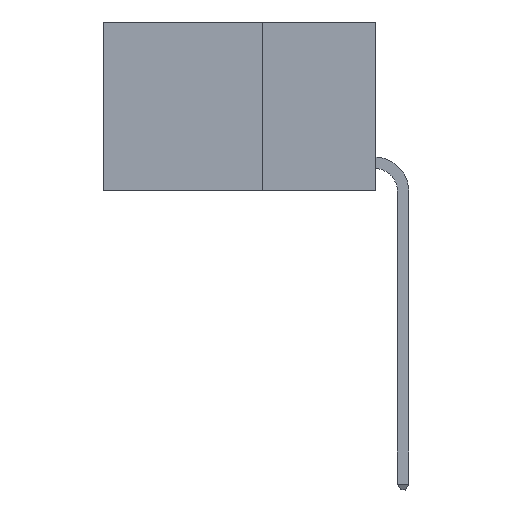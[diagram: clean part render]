
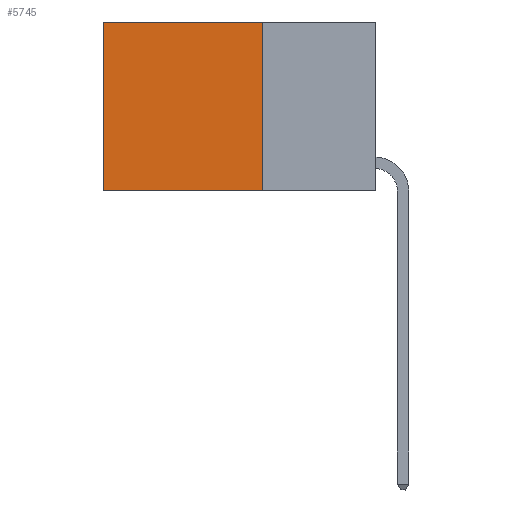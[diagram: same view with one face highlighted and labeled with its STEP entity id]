
A CAD part, left-side view. The second image highlights one B-rep face of the part: STEP entity #5745.
In plain terms, the highlighted planar face has unit normal (-1, 0, 0).
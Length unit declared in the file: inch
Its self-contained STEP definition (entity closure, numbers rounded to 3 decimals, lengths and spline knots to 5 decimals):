
#638 = CARTESIAN_POINT ( 'NONE',  ( 0.2625, 0.6, -0.37 ) ) ;
#828 = VECTOR ( 'NONE', #23020, 39.37008 ) ;
#937 = DIRECTION ( 'NONE',  ( 1., 0., 0. ) ) ;
#1519 = ORIENTED_EDGE ( 'NONE', *, *, #14590, .T. ) ;
#1627 = CARTESIAN_POINT ( 'NONE',  ( 0.2625, 0.25, 0. ) ) ;
#3688 = CARTESIAN_POINT ( 'NONE',  ( 0.2625, 0.25, 0. ) ) ;
#4303 = VECTOR ( 'NONE', #25474, 39.37008 ) ;
#4760 = EDGE_CURVE ( 'NONE', #25653, #25745, #23488, .T. ) ;
#5031 = DIRECTION ( 'NONE',  ( 0., 0., -1. ) ) ;
#5745 = ADVANCED_FACE ( 'NONE', ( #12976 ), #11008, .F. ) ;
#6198 = VERTEX_POINT ( 'NONE', #3688 ) ;
#7542 = CARTESIAN_POINT ( 'NONE',  ( 0.2625, 0.6, 0. ) ) ;
#8043 = VECTOR ( 'NONE', #16398, 39.37008 ) ;
#8261 = EDGE_CURVE ( 'NONE', #6198, #25653, #24998, .T. ) ;
#8448 = EDGE_CURVE ( 'NONE', #6198, #22909, #19741, .T. ) ;
#9805 = DIRECTION ( 'NONE',  ( 0., 0., -1. ) ) ;
#11008 = PLANE ( 'NONE',  #14078 ) ;
#12976 = FACE_OUTER_BOUND ( 'NONE', #14661, .T. ) ;
#13114 = ORIENTED_EDGE ( 'NONE', *, *, #8448, .T. ) ;
#13329 = CARTESIAN_POINT ( 'NONE',  ( 0.2625, 0.6, 0. ) ) ;
#14078 = AXIS2_PLACEMENT_3D ( 'NONE', #14698, #937, #5031 ) ;
#14590 = EDGE_CURVE ( 'NONE', #22909, #25745, #25600, .T. ) ;
#14661 = EDGE_LOOP ( 'NONE', ( #1519, #25498, #24419, #13114 ) ) ;
#14698 = CARTESIAN_POINT ( 'NONE',  ( 0.2625, 0.25, 0. ) ) ;
#15005 = CARTESIAN_POINT ( 'NONE',  ( 0.2625, 0.25, 0. ) ) ;
#15882 = CARTESIAN_POINT ( 'NONE',  ( 0.2625, 0.25, -0.37 ) ) ;
#16398 = DIRECTION ( 'NONE',  ( 0., 1., 0. ) ) ;
#17325 = CARTESIAN_POINT ( 'NONE',  ( 0.2625, 0.25, -0.37 ) ) ;
#19741 = LINE ( 'NONE', #1627, #8043 ) ;
#22909 = VERTEX_POINT ( 'NONE', #13329 ) ;
#23020 = DIRECTION ( 'NONE',  ( 0., 0., -1. ) ) ;
#23195 = VECTOR ( 'NONE', #9805, 39.37008 ) ;
#23488 = LINE ( 'NONE', #17325, #4303 ) ;
#24419 = ORIENTED_EDGE ( 'NONE', *, *, #8261, .F. ) ;
#24998 = LINE ( 'NONE', #15005, #828 ) ;
#25474 = DIRECTION ( 'NONE',  ( 0., 1., 0. ) ) ;
#25498 = ORIENTED_EDGE ( 'NONE', *, *, #4760, .F. ) ;
#25600 = LINE ( 'NONE', #7542, #23195 ) ;
#25653 = VERTEX_POINT ( 'NONE', #15882 ) ;
#25745 = VERTEX_POINT ( 'NONE', #638 ) ;
